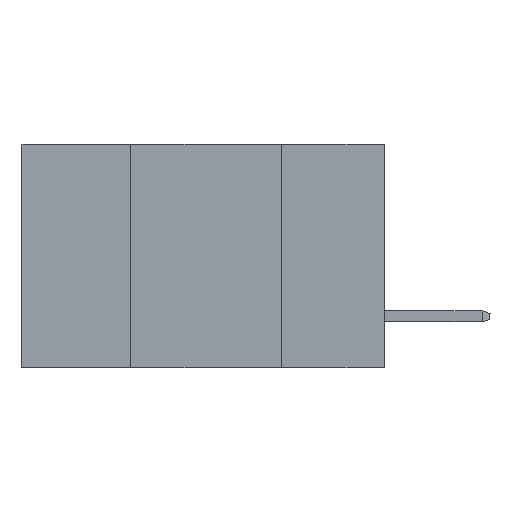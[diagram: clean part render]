
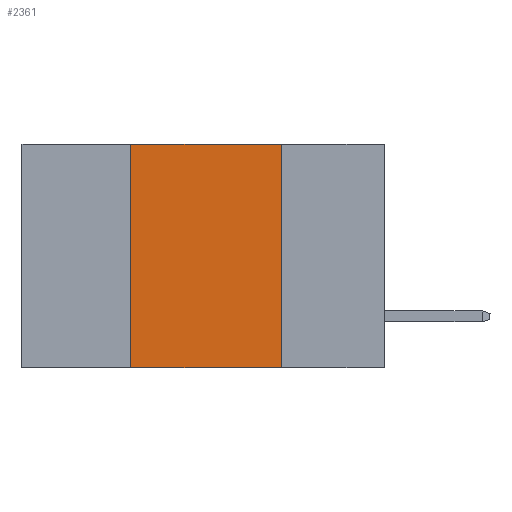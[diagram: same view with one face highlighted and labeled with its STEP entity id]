
A CAD part, left-side view. The second image highlights one B-rep face of the part: STEP entity #2361.
In plain terms, the highlighted planar face has unit normal (-1, 0, 0).
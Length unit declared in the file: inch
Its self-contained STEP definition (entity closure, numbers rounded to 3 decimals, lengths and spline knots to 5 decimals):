
#303 = CARTESIAN_POINT ( 'NONE',  ( 0., 0.17, -0.37 ) ) ;
#796 = CARTESIAN_POINT ( 'NONE',  ( 0., 0.42, 0. ) ) ;
#1125 = FACE_OUTER_BOUND ( 'NONE', #3924, .T. ) ;
#1595 = CARTESIAN_POINT ( 'NONE',  ( 0., 0.6, -0.37 ) ) ;
#1772 = CARTESIAN_POINT ( 'NONE',  ( 0., 0.6, 0. ) ) ;
#2075 = VERTEX_POINT ( 'NONE', #4337 ) ;
#2361 = ADVANCED_FACE ( 'NONE', ( #1125 ), #3299, .F. ) ;
#2406 = DIRECTION ( 'NONE',  ( 0., 0., -1. ) ) ;
#2509 = VECTOR ( 'NONE', #2406, 39.37008 ) ;
#2829 = VECTOR ( 'NONE', #5577, 39.37008 ) ;
#3086 = VERTEX_POINT ( 'NONE', #6379 ) ;
#3105 = DIRECTION ( 'NONE',  ( 0., -1., 0. ) ) ;
#3261 = LINE ( 'NONE', #1595, #9750 ) ;
#3299 = PLANE ( 'NONE',  #7302 ) ;
#3495 = VECTOR ( 'NONE', #8320, 39.37008 ) ;
#3924 = EDGE_LOOP ( 'NONE', ( #6777, #7632, #4367, #9366 ) ) ;
#4337 = CARTESIAN_POINT ( 'NONE',  ( 0., 0.42, -0.37 ) ) ;
#4367 = ORIENTED_EDGE ( 'NONE', *, *, #6870, .F. ) ;
#4645 = CARTESIAN_POINT ( 'NONE',  ( 0., 0.42, -0.37 ) ) ;
#4718 = LINE ( 'NONE', #9490, #2509 ) ;
#5395 = EDGE_CURVE ( 'NONE', #5980, #3086, #8843, .T. ) ;
#5577 = DIRECTION ( 'NONE',  ( 0., 0., 1. ) ) ;
#5832 = DIRECTION ( 'NONE',  ( 1., 0., 0. ) ) ;
#5980 = VERTEX_POINT ( 'NONE', #796 ) ;
#6379 = CARTESIAN_POINT ( 'NONE',  ( 0., 0.17, 0. ) ) ;
#6777 = ORIENTED_EDGE ( 'NONE', *, *, #7265, .F. ) ;
#6826 = EDGE_CURVE ( 'NONE', #2075, #9401, #3261, .T. ) ;
#6870 = EDGE_CURVE ( 'NONE', #2075, #5980, #10126, .T. ) ;
#7265 = EDGE_CURVE ( 'NONE', #3086, #9401, #4718, .T. ) ;
#7302 = AXIS2_PLACEMENT_3D ( 'NONE', #8094, #5832, #8981 ) ;
#7632 = ORIENTED_EDGE ( 'NONE', *, *, #5395, .F. ) ;
#8094 = CARTESIAN_POINT ( 'NONE',  ( 0., 0.6, 0. ) ) ;
#8320 = DIRECTION ( 'NONE',  ( 0., -1., 0. ) ) ;
#8843 = LINE ( 'NONE', #1772, #3495 ) ;
#8981 = DIRECTION ( 'NONE',  ( 0., 0., -1. ) ) ;
#9366 = ORIENTED_EDGE ( 'NONE', *, *, #6826, .T. ) ;
#9401 = VERTEX_POINT ( 'NONE', #303 ) ;
#9490 = CARTESIAN_POINT ( 'NONE',  ( 0., 0.17, -0.37 ) ) ;
#9750 = VECTOR ( 'NONE', #3105, 39.37008 ) ;
#10126 = LINE ( 'NONE', #4645, #2829 ) ;
